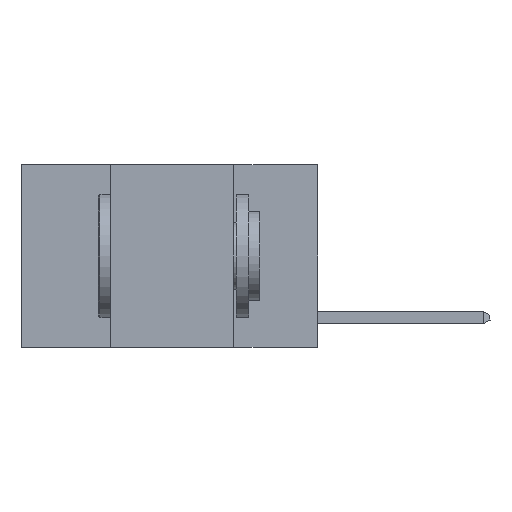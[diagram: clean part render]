
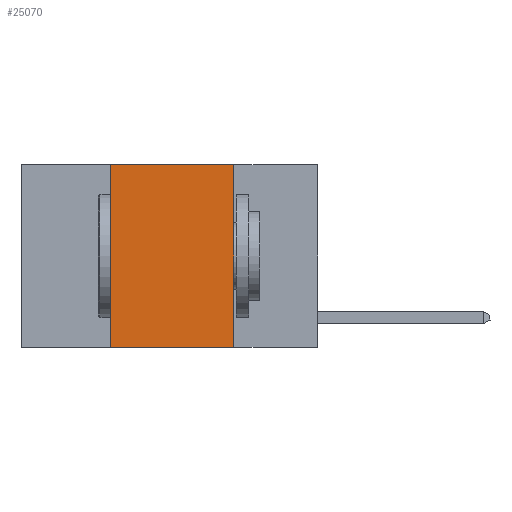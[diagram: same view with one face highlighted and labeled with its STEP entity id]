
A CAD part, left-side view. The second image highlights one B-rep face of the part: STEP entity #25070.
In plain terms, the highlighted planar face has unit normal (-1, 0, 0).
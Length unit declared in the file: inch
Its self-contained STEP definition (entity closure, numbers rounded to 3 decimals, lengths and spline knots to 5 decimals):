
#321 = CARTESIAN_POINT ( 'NONE',  ( 0., 0.42, -0.37 ) ) ;
#395 = CARTESIAN_POINT ( 'NONE',  ( 0., 0.6, -0.37 ) ) ;
#1106 = ORIENTED_EDGE ( 'NONE', *, *, #7928, .T. ) ;
#1190 = LINE ( 'NONE', #1620, #16741 ) ;
#1594 = DIRECTION ( 'NONE',  ( 0., -1., 0. ) ) ;
#1620 = CARTESIAN_POINT ( 'NONE',  ( 0., 0.6, 0. ) ) ;
#1766 = CARTESIAN_POINT ( 'NONE',  ( 0., 0.17, -0.37 ) ) ;
#2196 = EDGE_CURVE ( 'NONE', #9911, #23154, #1190, .T. ) ;
#3947 = PLANE ( 'NONE',  #20026 ) ;
#5993 = CARTESIAN_POINT ( 'NONE',  ( 0., 0.6, 0. ) ) ;
#6846 = ORIENTED_EDGE ( 'NONE', *, *, #13282, .F. ) ;
#7928 = EDGE_CURVE ( 'NONE', #19364, #15544, #24434, .T. ) ;
#8037 = DIRECTION ( 'NONE',  ( 0., 0., -1. ) ) ;
#8072 = LINE ( 'NONE', #21774, #24317 ) ;
#9911 = VERTEX_POINT ( 'NONE', #23804 ) ;
#10049 = ORIENTED_EDGE ( 'NONE', *, *, #16525, .F. ) ;
#10136 = VECTOR ( 'NONE', #20950, 39.37008 ) ;
#12241 = ORIENTED_EDGE ( 'NONE', *, *, #2196, .F. ) ;
#13282 = EDGE_CURVE ( 'NONE', #23154, #15544, #8072, .T. ) ;
#13569 = DIRECTION ( 'NONE',  ( 0., 0., -1. ) ) ;
#14245 = LINE ( 'NONE', #19037, #10136 ) ;
#15544 = VERTEX_POINT ( 'NONE', #1766 ) ;
#16525 = EDGE_CURVE ( 'NONE', #19364, #9911, #14245, .T. ) ;
#16741 = VECTOR ( 'NONE', #1594, 39.37008 ) ;
#18958 = VECTOR ( 'NONE', #24812, 39.37008 ) ;
#19037 = CARTESIAN_POINT ( 'NONE',  ( 0., 0.42, 0. ) ) ;
#19085 = FACE_OUTER_BOUND ( 'NONE', #25023, .T. ) ;
#19364 = VERTEX_POINT ( 'NONE', #321 ) ;
#20026 = AXIS2_PLACEMENT_3D ( 'NONE', #5993, #20208, #8037 ) ;
#20208 = DIRECTION ( 'NONE',  ( 1., 0., 0. ) ) ;
#20950 = DIRECTION ( 'NONE',  ( 0., 0., 1. ) ) ;
#21774 = CARTESIAN_POINT ( 'NONE',  ( 0., 0.17, 0. ) ) ;
#23154 = VERTEX_POINT ( 'NONE', #24322 ) ;
#23804 = CARTESIAN_POINT ( 'NONE',  ( 0., 0.42, 0. ) ) ;
#24317 = VECTOR ( 'NONE', #13569, 39.37008 ) ;
#24322 = CARTESIAN_POINT ( 'NONE',  ( 0., 0.17, 0. ) ) ;
#24434 = LINE ( 'NONE', #395, #18958 ) ;
#24812 = DIRECTION ( 'NONE',  ( 0., -1., 0. ) ) ;
#25023 = EDGE_LOOP ( 'NONE', ( #6846, #12241, #10049, #1106 ) ) ;
#25070 = ADVANCED_FACE ( 'NONE', ( #19085 ), #3947, .F. ) ;
